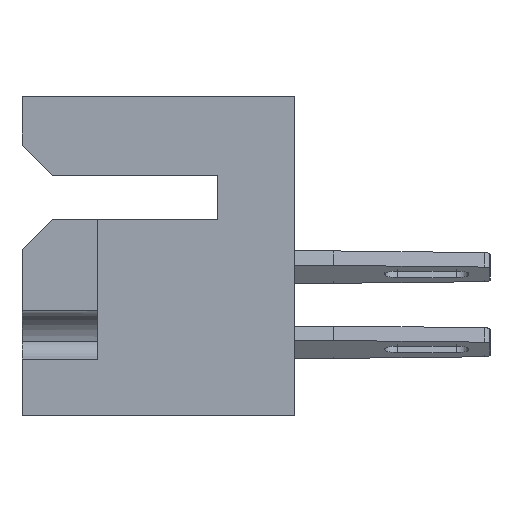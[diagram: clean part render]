
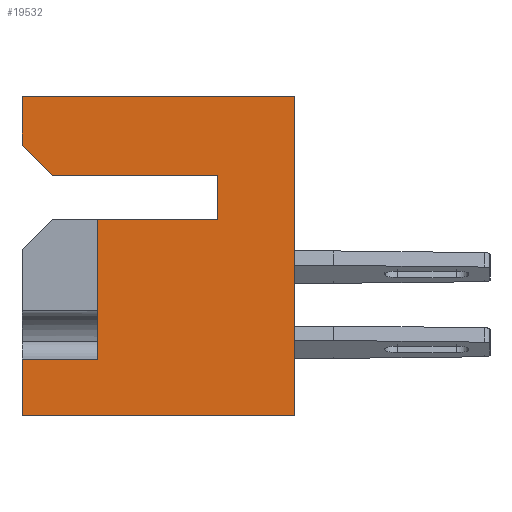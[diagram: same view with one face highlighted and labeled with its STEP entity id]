
A CAD part, left-side view. The second image highlights one B-rep face of the part: STEP entity #19532.
In plain terms, the highlighted planar face has unit normal (-1, 0, 0).
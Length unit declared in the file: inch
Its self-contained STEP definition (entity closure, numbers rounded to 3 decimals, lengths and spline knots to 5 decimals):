
#530 = VECTOR ( 'NONE', #11698, 39.37008 ) ;
#568 = CARTESIAN_POINT ( 'NONE',  ( 0., 0.328, -0.437 ) ) ;
#850 = ORIENTED_EDGE ( 'NONE', *, *, #14169, .F. ) ;
#1018 = EDGE_CURVE ( 'NONE', #17379, #7703, #3516, .T. ) ;
#1021 = ORIENTED_EDGE ( 'NONE', *, *, #14083, .F. ) ;
#1274 = EDGE_CURVE ( 'NONE', #5012, #9012, #16653, .T. ) ;
#1385 = ORIENTED_EDGE ( 'NONE', *, *, #6375, .T. ) ;
#1832 = VECTOR ( 'NONE', #12286, 39.37008 ) ;
#2006 = CARTESIAN_POINT ( 'NONE',  ( 0., 0.328, -0.437 ) ) ;
#2207 = CARTESIAN_POINT ( 'NONE',  ( 0., 0.453, -0.531 ) ) ;
#2418 = EDGE_CURVE ( 'NONE', #12957, #17379, #15914, .T. ) ;
#2725 = LINE ( 'NONE', #2207, #11510 ) ;
#2855 = DIRECTION ( 'NONE',  ( 0., 1., 0. ) ) ;
#3204 = PLANE ( 'NONE',  #17359 ) ;
#3516 = LINE ( 'NONE', #13518, #11570 ) ;
#4027 = VECTOR ( 'NONE', #2855, 39.37008 ) ;
#4083 = CARTESIAN_POINT ( 'NONE',  ( 0., 0.453, 0. ) ) ;
#4177 = CARTESIAN_POINT ( 'NONE',  ( 0., 0.453, -0.437 ) ) ;
#4197 = DIRECTION ( 'NONE',  ( 0., -1., 0. ) ) ;
#4746 = CARTESIAN_POINT ( 'NONE',  ( 0., 0.128, -0.205 ) ) ;
#4780 = DIRECTION ( 'NONE',  ( 0., 0., -1. ) ) ;
#5012 = VERTEX_POINT ( 'NONE', #18825 ) ;
#5205 = CARTESIAN_POINT ( 'NONE',  ( 0., 0.328, -0.205 ) ) ;
#5240 = ORIENTED_EDGE ( 'NONE', *, *, #8611, .F. ) ;
#5301 = DIRECTION ( 'NONE',  ( 0., 1., 0. ) ) ;
#5471 = ORIENTED_EDGE ( 'NONE', *, *, #20110, .F. ) ;
#6185 = VECTOR ( 'NONE', #10253, 39.37008 ) ;
#6326 = CARTESIAN_POINT ( 'NONE',  ( 0., 0.403, -0.131 ) ) ;
#6375 = EDGE_CURVE ( 'NONE', #10564, #9134, #19353, .T. ) ;
#6439 = DIRECTION ( 'NONE',  ( 0., 0., 1. ) ) ;
#6764 = VECTOR ( 'NONE', #7774, 39.37008 ) ;
#6961 = VECTOR ( 'NONE', #8371, 39.37008 ) ;
#6985 = DIRECTION ( 'NONE',  ( 0., -1., 0. ) ) ;
#7703 = VERTEX_POINT ( 'NONE', #10383 ) ;
#7774 = DIRECTION ( 'NONE',  ( 0., -0.707, -0.707 ) ) ;
#7941 = CARTESIAN_POINT ( 'NONE',  ( 0., 0.453, 0. ) ) ;
#8371 = DIRECTION ( 'NONE',  ( 0., 0., 1. ) ) ;
#8611 = EDGE_CURVE ( 'NONE', #12004, #16708, #14496, .T. ) ;
#8635 = CARTESIAN_POINT ( 'NONE',  ( 0., 0.453, 0. ) ) ;
#8689 = CARTESIAN_POINT ( 'NONE',  ( 0., 0., 0. ) ) ;
#9012 = VERTEX_POINT ( 'NONE', #5205 ) ;
#9134 = VERTEX_POINT ( 'NONE', #4177 ) ;
#9172 = LINE ( 'NONE', #14059, #1832 ) ;
#9478 = EDGE_CURVE ( 'NONE', #13018, #7703, #13245, .T. ) ;
#9690 = CARTESIAN_POINT ( 'NONE',  ( 0., 0.403, -0.131 ) ) ;
#9972 = CARTESIAN_POINT ( 'NONE',  ( 0., 0.128, -0.131 ) ) ;
#10253 = DIRECTION ( 'NONE',  ( 0., 0., 1. ) ) ;
#10383 = CARTESIAN_POINT ( 'NONE',  ( 0., 0., 0. ) ) ;
#10564 = VERTEX_POINT ( 'NONE', #568 ) ;
#10584 = ORIENTED_EDGE ( 'NONE', *, *, #12906, .T. ) ;
#10636 = LINE ( 'NONE', #11100, #6961 ) ;
#10822 = DIRECTION ( 'NONE',  ( 0., 1., 0. ) ) ;
#11100 = CARTESIAN_POINT ( 'NONE',  ( 0., 0.128, -0.131 ) ) ;
#11364 = VECTOR ( 'NONE', #5301, 39.37008 ) ;
#11510 = VECTOR ( 'NONE', #6985, 39.37008 ) ;
#11570 = VECTOR ( 'NONE', #4197, 39.37008 ) ;
#11698 = DIRECTION ( 'NONE',  ( 0., 0., 1. ) ) ;
#12004 = VERTEX_POINT ( 'NONE', #9972 ) ;
#12286 = DIRECTION ( 'NONE',  ( 0., 0., 1. ) ) ;
#12906 = EDGE_CURVE ( 'NONE', #12957, #16708, #19372, .T. ) ;
#12957 = VERTEX_POINT ( 'NONE', #15570 ) ;
#13018 = VERTEX_POINT ( 'NONE', #15766 ) ;
#13245 = LINE ( 'NONE', #8689, #6185 ) ;
#13342 = ORIENTED_EDGE ( 'NONE', *, *, #1018, .F. ) ;
#13488 = ORIENTED_EDGE ( 'NONE', *, *, #15754, .T. ) ;
#13518 = CARTESIAN_POINT ( 'NONE',  ( 0., 0.453, 0. ) ) ;
#14059 = CARTESIAN_POINT ( 'NONE',  ( 0., 0.328, -0.205 ) ) ;
#14083 = EDGE_CURVE ( 'NONE', #10564, #9012, #9172, .T. ) ;
#14106 = DIRECTION ( 'NONE',  ( 1., 0., 0. ) ) ;
#14147 = ORIENTED_EDGE ( 'NONE', *, *, #2418, .F. ) ;
#14153 = ORIENTED_EDGE ( 'NONE', *, *, #9478, .T. ) ;
#14169 = EDGE_CURVE ( 'NONE', #18681, #9134, #15974, .T. ) ;
#14496 = LINE ( 'NONE', #16814, #4027 ) ;
#14924 = EDGE_LOOP ( 'NONE', ( #1385, #850, #13488, #14153, #13342, #14147, #10584, #5240, #5471, #19762, #1021 ) ) ;
#15570 = CARTESIAN_POINT ( 'NONE',  ( 0., 0.453, -0.081 ) ) ;
#15754 = EDGE_CURVE ( 'NONE', #18681, #13018, #2725, .T. ) ;
#15766 = CARTESIAN_POINT ( 'NONE',  ( 0., 0., -0.531 ) ) ;
#15914 = LINE ( 'NONE', #4083, #530 ) ;
#15974 = LINE ( 'NONE', #7941, #17926 ) ;
#16653 = LINE ( 'NONE', #4746, #18127 ) ;
#16708 = VERTEX_POINT ( 'NONE', #9690 ) ;
#16814 = CARTESIAN_POINT ( 'NONE',  ( 0., 0.128, -0.131 ) ) ;
#17359 = AXIS2_PLACEMENT_3D ( 'NONE', #20134, #14106, #4780 ) ;
#17379 = VERTEX_POINT ( 'NONE', #8635 ) ;
#17926 = VECTOR ( 'NONE', #6439, 39.37008 ) ;
#18043 = CARTESIAN_POINT ( 'NONE',  ( 0., 0.453, -0.531 ) ) ;
#18127 = VECTOR ( 'NONE', #10822, 39.37008 ) ;
#18681 = VERTEX_POINT ( 'NONE', #18043 ) ;
#18825 = CARTESIAN_POINT ( 'NONE',  ( 0., 0.128, -0.205 ) ) ;
#19353 = LINE ( 'NONE', #2006, #11364 ) ;
#19372 = LINE ( 'NONE', #6326, #6764 ) ;
#19532 = ADVANCED_FACE ( 'NONE', ( #19631 ), #3204, .F. ) ;
#19631 = FACE_OUTER_BOUND ( 'NONE', #14924, .T. ) ;
#19762 = ORIENTED_EDGE ( 'NONE', *, *, #1274, .T. ) ;
#20110 = EDGE_CURVE ( 'NONE', #5012, #12004, #10636, .T. ) ;
#20134 = CARTESIAN_POINT ( 'NONE',  ( 0., 0.453, 0. ) ) ;
